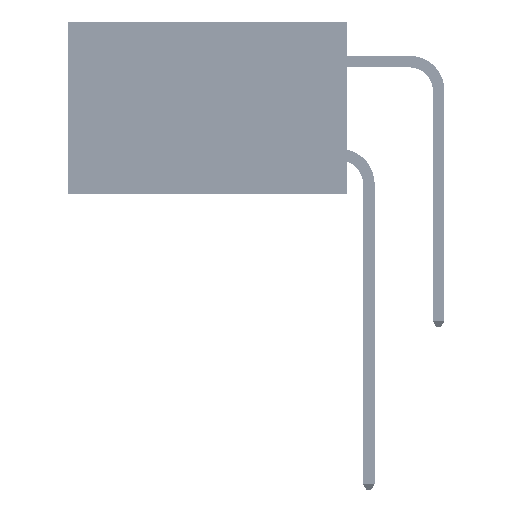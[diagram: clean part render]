
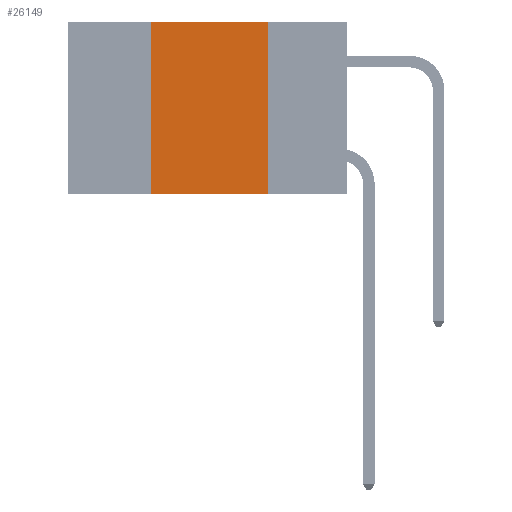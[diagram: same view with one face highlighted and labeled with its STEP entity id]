
A CAD part, left-side view. The second image highlights one B-rep face of the part: STEP entity #26149.
In plain terms, the highlighted planar face has unit normal (-1, 0, 0).
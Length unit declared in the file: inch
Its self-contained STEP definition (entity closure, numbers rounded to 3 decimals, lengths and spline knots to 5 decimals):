
#155 = VERTEX_POINT ( 'NONE', #25482 ) ;
#1693 = ORIENTED_EDGE ( 'NONE', *, *, #47155, .F. ) ;
#3812 = VECTOR ( 'NONE', #43352, 39.37008 ) ;
#6276 = VERTEX_POINT ( 'NONE', #31602 ) ;
#9723 = VERTEX_POINT ( 'NONE', #42107 ) ;
#10722 = LINE ( 'NONE', #22655, #30139 ) ;
#11093 = EDGE_CURVE ( 'NONE', #155, #24050, #14218, .T. ) ;
#11116 = PLANE ( 'NONE',  #14404 ) ;
#11278 = DIRECTION ( 'NONE',  ( 1., 0., 0. ) ) ;
#12356 = CARTESIAN_POINT ( 'NONE',  ( 0., 0.6, -0.37 ) ) ;
#14218 = LINE ( 'NONE', #12356, #3812 ) ;
#14404 = AXIS2_PLACEMENT_3D ( 'NONE', #15013, #11278, #38375 ) ;
#14847 = VECTOR ( 'NONE', #17039, 39.37008 ) ;
#15013 = CARTESIAN_POINT ( 'NONE',  ( 0., 0.6, 0. ) ) ;
#15696 = VECTOR ( 'NONE', #17616, 39.37008 ) ;
#17039 = DIRECTION ( 'NONE',  ( 0., 0., 1. ) ) ;
#17600 = ORIENTED_EDGE ( 'NONE', *, *, #25521, .F. ) ;
#17616 = DIRECTION ( 'NONE',  ( 0., -1., 0. ) ) ;
#22283 = CARTESIAN_POINT ( 'NONE',  ( 0., 0.17, -0.37 ) ) ;
#22655 = CARTESIAN_POINT ( 'NONE',  ( 0., 0.17, 0. ) ) ;
#24050 = VERTEX_POINT ( 'NONE', #22283 ) ;
#25222 = LINE ( 'NONE', #36322, #14847 ) ;
#25482 = CARTESIAN_POINT ( 'NONE',  ( 0., 0.42, -0.37 ) ) ;
#25521 = EDGE_CURVE ( 'NONE', #6276, #24050, #10722, .T. ) ;
#26135 = ORIENTED_EDGE ( 'NONE', *, *, #11093, .T. ) ;
#26149 = ADVANCED_FACE ( 'NONE', ( #42146 ), #11116, .F. ) ;
#26483 = EDGE_CURVE ( 'NONE', #155, #9723, #25222, .T. ) ;
#30139 = VECTOR ( 'NONE', #34439, 39.37008 ) ;
#31602 = CARTESIAN_POINT ( 'NONE',  ( 0., 0.17, 0. ) ) ;
#32721 = ORIENTED_EDGE ( 'NONE', *, *, #26483, .F. ) ;
#34439 = DIRECTION ( 'NONE',  ( 0., 0., -1. ) ) ;
#36322 = CARTESIAN_POINT ( 'NONE',  ( 0., 0.42, 0. ) ) ;
#36879 = CARTESIAN_POINT ( 'NONE',  ( 0., 0.6, 0. ) ) ;
#38375 = DIRECTION ( 'NONE',  ( 0., 0., -1. ) ) ;
#39923 = LINE ( 'NONE', #36879, #15696 ) ;
#40880 = EDGE_LOOP ( 'NONE', ( #17600, #1693, #32721, #26135 ) ) ;
#42107 = CARTESIAN_POINT ( 'NONE',  ( 0., 0.42, 0. ) ) ;
#42146 = FACE_OUTER_BOUND ( 'NONE', #40880, .T. ) ;
#43352 = DIRECTION ( 'NONE',  ( 0., -1., 0. ) ) ;
#47155 = EDGE_CURVE ( 'NONE', #9723, #6276, #39923, .T. ) ;
